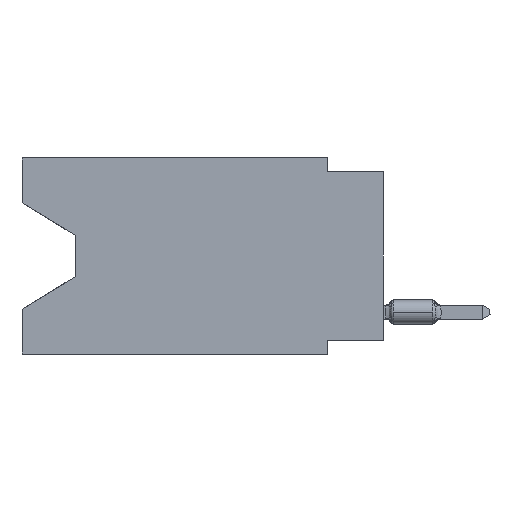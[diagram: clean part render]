
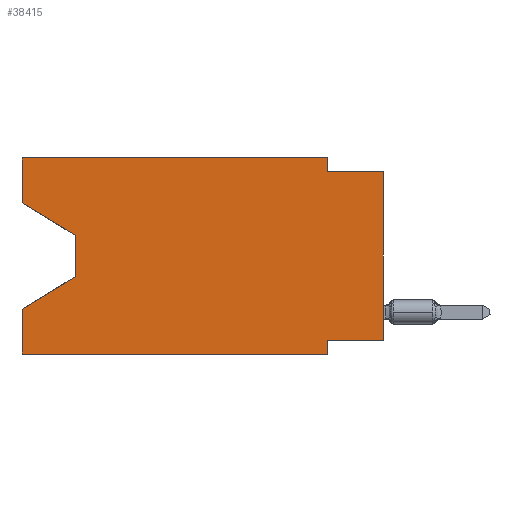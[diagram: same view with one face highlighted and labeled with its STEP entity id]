
A CAD part, left-side view. The second image highlights one B-rep face of the part: STEP entity #38415.
In plain terms, the highlighted planar face has unit normal (-1, 0, 0).
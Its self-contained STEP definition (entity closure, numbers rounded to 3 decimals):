
#444 = DIRECTION ( 'NONE',  ( 0., 1., 0. ) ) ;
#720 = CARTESIAN_POINT ( 'NONE',  ( 0., 2.54, -0.635 ) ) ;
#1601 = ORIENTED_EDGE ( 'NONE', *, *, #10941, .F. ) ;
#1767 = DIRECTION ( 'NONE',  ( 0., -0.855, -0.519 ) ) ;
#2026 = PLANE ( 'NONE',  #3939 ) ;
#2108 = VECTOR ( 'NONE', #32038, 1000. ) ;
#2437 = VECTOR ( 'NONE', #19960, 1000. ) ;
#2802 = ORIENTED_EDGE ( 'NONE', *, *, #13540, .T. ) ;
#3384 = DIRECTION ( 'NONE',  ( 0., -1., 0. ) ) ;
#3745 = DIRECTION ( 'NONE',  ( 0., -1., 0. ) ) ;
#3905 = DIRECTION ( 'NONE',  ( 0., 0., -1. ) ) ;
#3939 = AXIS2_PLACEMENT_3D ( 'NONE', #15031, #28221, #28009 ) ;
#4487 = ORIENTED_EDGE ( 'NONE', *, *, #13943, .T. ) ;
#4586 = CARTESIAN_POINT ( 'NONE',  ( 0., 2.54, 0. ) ) ;
#5225 = FACE_OUTER_BOUND ( 'NONE', #37560, .T. ) ;
#7896 = VECTOR ( 'NONE', #9531, 1000. ) ;
#7901 = VERTEX_POINT ( 'NONE', #13878 ) ;
#8109 = ORIENTED_EDGE ( 'NONE', *, *, #27045, .F. ) ;
#8832 = LINE ( 'NONE', #17229, #34661 ) ;
#8921 = ORIENTED_EDGE ( 'NONE', *, *, #26247, .F. ) ;
#8950 = ORIENTED_EDGE ( 'NONE', *, *, #12051, .T. ) ;
#9028 = CARTESIAN_POINT ( 'NONE',  ( 0., 0., -8.255 ) ) ;
#9531 = DIRECTION ( 'NONE',  ( 0., 0., -1. ) ) ;
#9886 = CARTESIAN_POINT ( 'NONE',  ( 0., 2.54, 0. ) ) ;
#10575 = CARTESIAN_POINT ( 'NONE',  ( 0., 0., 0. ) ) ;
#10835 = DIRECTION ( 'NONE',  ( 0., 0., 1. ) ) ;
#10941 = EDGE_CURVE ( 'NONE', #23711, #40913, #21090, .T. ) ;
#12051 = EDGE_CURVE ( 'NONE', #30548, #40913, #32981, .T. ) ;
#12682 = VERTEX_POINT ( 'NONE', #24625 ) ;
#12957 = VERTEX_POINT ( 'NONE', #720 ) ;
#13540 = EDGE_CURVE ( 'NONE', #12682, #7901, #37882, .T. ) ;
#13878 = CARTESIAN_POINT ( 'NONE',  ( 0., 13.97, -5.385 ) ) ;
#13943 = EDGE_CURVE ( 'NONE', #21927, #28336, #27174, .T. ) ;
#14031 = CARTESIAN_POINT ( 'NONE',  ( 0., 16.383, 0. ) ) ;
#14899 = CARTESIAN_POINT ( 'NONE',  ( 0., 2.54, -8.89 ) ) ;
#15031 = CARTESIAN_POINT ( 'NONE',  ( 0., 16.383, 0. ) ) ;
#16215 = ORIENTED_EDGE ( 'NONE', *, *, #37785, .F. ) ;
#17229 = CARTESIAN_POINT ( 'NONE',  ( 0., 16.383, 0. ) ) ;
#17611 = CARTESIAN_POINT ( 'NONE',  ( 0., 16.383, -6.852 ) ) ;
#17761 = LINE ( 'NONE', #40124, #28660 ) ;
#18009 = CARTESIAN_POINT ( 'NONE',  ( 0., 16.383, 0. ) ) ;
#18523 = VERTEX_POINT ( 'NONE', #38829 ) ;
#19960 = DIRECTION ( 'NONE',  ( 0., 0., 1. ) ) ;
#21090 = LINE ( 'NONE', #14899, #30260 ) ;
#21588 = CARTESIAN_POINT ( 'NONE',  ( 0., 0., -0.635 ) ) ;
#21701 = CARTESIAN_POINT ( 'NONE',  ( 0., 13.97, -3.505 ) ) ;
#21927 = VERTEX_POINT ( 'NONE', #9028 ) ;
#22678 = CARTESIAN_POINT ( 'NONE',  ( 0., 13.97, -5.385 ) ) ;
#23246 = LINE ( 'NONE', #23882, #34145 ) ;
#23353 = LINE ( 'NONE', #39744, #31332 ) ;
#23711 = VERTEX_POINT ( 'NONE', #25639 ) ;
#23857 = LINE ( 'NONE', #36855, #25526 ) ;
#23882 = CARTESIAN_POINT ( 'NONE',  ( 0., 0., -8.255 ) ) ;
#24625 = CARTESIAN_POINT ( 'NONE',  ( 0., 13.97, -3.505 ) ) ;
#24728 = VERTEX_POINT ( 'NONE', #4586 ) ;
#25526 = VECTOR ( 'NONE', #30020, 1000. ) ;
#25639 = CARTESIAN_POINT ( 'NONE',  ( 0., 2.54, -8.255 ) ) ;
#26247 = EDGE_CURVE ( 'NONE', #30548, #38170, #33401, .T. ) ;
#26658 = EDGE_CURVE ( 'NONE', #41932, #24728, #23353, .T. ) ;
#26929 = EDGE_CURVE ( 'NONE', #7901, #38170, #31835, .T. ) ;
#27045 = EDGE_CURVE ( 'NONE', #24728, #12957, #39696, .T. ) ;
#27174 = LINE ( 'NONE', #10575, #2437 ) ;
#27198 = EDGE_CURVE ( 'NONE', #18523, #12682, #17761, .T. ) ;
#27219 = DIRECTION ( 'NONE',  ( 0., 0., 1. ) ) ;
#28009 = DIRECTION ( 'NONE',  ( 0., 0., -1. ) ) ;
#28221 = DIRECTION ( 'NONE',  ( 1., 0., 0. ) ) ;
#28336 = VERTEX_POINT ( 'NONE', #21588 ) ;
#28660 = VECTOR ( 'NONE', #1767, 1000. ) ;
#29319 = ORIENTED_EDGE ( 'NONE', *, *, #26929, .T. ) ;
#29781 = ORIENTED_EDGE ( 'NONE', *, *, #26658, .F. ) ;
#30020 = DIRECTION ( 'NONE',  ( 0., -1., 0. ) ) ;
#30260 = VECTOR ( 'NONE', #40670, 1000. ) ;
#30353 = VECTOR ( 'NONE', #3384, 1000. ) ;
#30548 = VERTEX_POINT ( 'NONE', #39985 ) ;
#31332 = VECTOR ( 'NONE', #3745, 1000. ) ;
#31711 = EDGE_CURVE ( 'NONE', #12957, #28336, #23857, .T. ) ;
#31835 = LINE ( 'NONE', #22678, #2108 ) ;
#32038 = DIRECTION ( 'NONE',  ( 0., 0.855, -0.519 ) ) ;
#32819 = ORIENTED_EDGE ( 'NONE', *, *, #35158, .F. ) ;
#32981 = LINE ( 'NONE', #36405, #30353 ) ;
#33401 = LINE ( 'NONE', #14031, #37534 ) ;
#34145 = VECTOR ( 'NONE', #444, 1000. ) ;
#34562 = ORIENTED_EDGE ( 'NONE', *, *, #27198, .T. ) ;
#34661 = VECTOR ( 'NONE', #27219, 1000. ) ;
#35158 = EDGE_CURVE ( 'NONE', #18523, #41932, #8832, .T. ) ;
#35805 = CARTESIAN_POINT ( 'NONE',  ( 0., 2.54, -8.89 ) ) ;
#36405 = CARTESIAN_POINT ( 'NONE',  ( 0., 16.383, -8.89 ) ) ;
#36855 = CARTESIAN_POINT ( 'NONE',  ( 0., 0., -0.635 ) ) ;
#37526 = VECTOR ( 'NONE', #3905, 1000. ) ;
#37534 = VECTOR ( 'NONE', #10835, 1000. ) ;
#37560 = EDGE_LOOP ( 'NONE', ( #34562, #2802, #29319, #8921, #8950, #1601, #16215, #4487, #40780, #8109, #29781, #32819 ) ) ;
#37785 = EDGE_CURVE ( 'NONE', #21927, #23711, #23246, .T. ) ;
#37882 = LINE ( 'NONE', #21701, #7896 ) ;
#38170 = VERTEX_POINT ( 'NONE', #17611 ) ;
#38415 = ADVANCED_FACE ( 'NONE', ( #5225 ), #2026, .F. ) ;
#38829 = CARTESIAN_POINT ( 'NONE',  ( 0., 16.383, -2.038 ) ) ;
#39696 = LINE ( 'NONE', #9886, #37526 ) ;
#39744 = CARTESIAN_POINT ( 'NONE',  ( 0., 16.383, 0. ) ) ;
#39985 = CARTESIAN_POINT ( 'NONE',  ( 0., 16.383, -8.89 ) ) ;
#40124 = CARTESIAN_POINT ( 'NONE',  ( 0., 16.383, -2.038 ) ) ;
#40670 = DIRECTION ( 'NONE',  ( 0., 0., -1. ) ) ;
#40780 = ORIENTED_EDGE ( 'NONE', *, *, #31711, .F. ) ;
#40913 = VERTEX_POINT ( 'NONE', #35805 ) ;
#41932 = VERTEX_POINT ( 'NONE', #18009 ) ;
